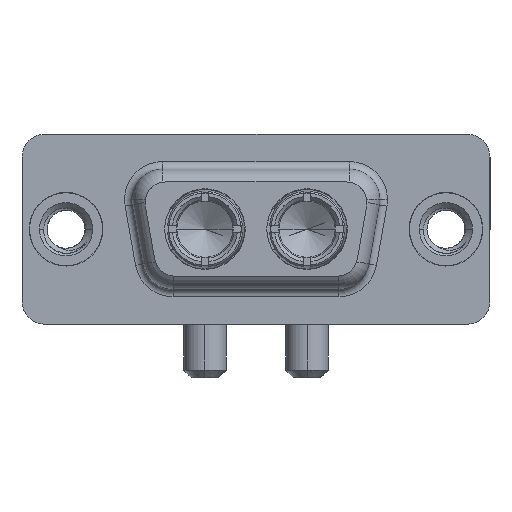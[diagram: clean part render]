
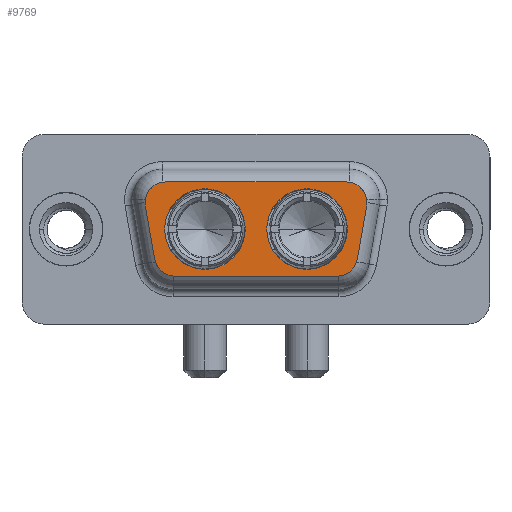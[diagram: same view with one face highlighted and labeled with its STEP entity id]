
A CAD part, top view. The second image highlights one B-rep face of the part: STEP entity #9769.
In plain terms, the highlighted planar face has unit normal (0, 0, 1).
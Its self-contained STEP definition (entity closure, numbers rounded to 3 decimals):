
#40 = DIRECTION ( 'NONE',  ( 0.174, -0.985, 0. ) ) ;
#42 = EDGE_CURVE ( 'NONE', #5957, #405, #10001, .T. ) ;
#180 = DIRECTION ( 'NONE',  ( -1., 0., 0. ) ) ;
#302 = AXIS2_PLACEMENT_3D ( 'NONE', #5699, #8658, #4725 ) ;
#391 = AXIS2_PLACEMENT_3D ( 'NONE', #10388, #2899, #4603 ) ;
#405 = VERTEX_POINT ( 'NONE', #8874 ) ;
#406 = CARTESIAN_POINT ( 'NONE',  ( 5.838, -1.984, 6.2 ) ) ;
#421 = CARTESIAN_POINT ( 'NONE',  ( 6.49, 0., 6.2 ) ) ;
#430 = VERTEX_POINT ( 'NONE', #421 ) ;
#628 = DIRECTION ( 'NONE',  ( -1., 0., 0. ) ) ;
#633 = EDGE_CURVE ( 'NONE', #10722, #5175, #7628, .T. ) ;
#653 = CARTESIAN_POINT ( 'NONE',  ( 17.833, -3.1, 6.2 ) ) ;
#724 = ORIENTED_EDGE ( 'NONE', *, *, #11435, .F. ) ;
#856 = CARTESIAN_POINT ( 'NONE',  ( 15.86, 0., 6.2 ) ) ;
#863 = VERTEX_POINT ( 'NONE', #6084 ) ;
#885 = VERTEX_POINT ( 'NONE', #406 ) ;
#1068 = DIRECTION ( 'NONE',  ( 0., 0., 1. ) ) ;
#1142 = VECTOR ( 'NONE', #3332, 1000. ) ;
#1339 = CIRCLE ( 'NONE', #9155, 1.35 ) ;
#1358 = ORIENTED_EDGE ( 'NONE', *, *, #3806, .T. ) ;
#1427 = LINE ( 'NONE', #10664, #9747 ) ;
#1580 = LINE ( 'NONE', #5340, #1142 ) ;
#1646 = DIRECTION ( 'NONE',  ( 1., 0., 0. ) ) ;
#1678 = CARTESIAN_POINT ( 'NONE',  ( 7.167, -1.75, 6.2 ) ) ;
#1778 = DIRECTION ( 'NONE',  ( 0., 0., 1. ) ) ;
#1855 = EDGE_CURVE ( 'NONE', #11892, #7952, #1427, .T. ) ;
#1967 = CARTESIAN_POINT ( 'NONE',  ( 7.167, -1.75, 6.2 ) ) ;
#1995 = ORIENTED_EDGE ( 'NONE', *, *, #9292, .T. ) ;
#2154 = ORIENTED_EDGE ( 'NONE', *, *, #11271, .F. ) ;
#2359 = AXIS2_PLACEMENT_3D ( 'NONE', #856, #1778, #2805 ) ;
#2431 = ORIENTED_EDGE ( 'NONE', *, *, #6789, .T. ) ;
#2529 = PLANE ( 'NONE',  #8586 ) ;
#2542 = CARTESIAN_POINT ( 'NONE',  ( 9.14, 0., 6.2 ) ) ;
#2555 = CARTESIAN_POINT ( 'NONE',  ( 6.55, 1.75, 6.2 ) ) ;
#2789 = ORIENTED_EDGE ( 'NONE', *, *, #1855, .T. ) ;
#2805 = DIRECTION ( 'NONE',  ( 1., 0., 0. ) ) ;
#2842 = ORIENTED_EDGE ( 'NONE', *, *, #633, .T. ) ;
#2899 = DIRECTION ( 'NONE',  ( 0., 0., 1. ) ) ;
#3009 = CARTESIAN_POINT ( 'NONE',  ( 18.45, 1.75, 6.2 ) ) ;
#3094 = CIRCLE ( 'NONE', #12130, 1.35 ) ;
#3165 = CARTESIAN_POINT ( 'NONE',  ( 5.2, 1.75, 6.2 ) ) ;
#3190 = EDGE_CURVE ( 'NONE', #10426, #430, #6930, .T. ) ;
#3332 = DIRECTION ( 'NONE',  ( 0.174, 0.985, 0. ) ) ;
#3621 = ORIENTED_EDGE ( 'NONE', *, *, #6040, .T. ) ;
#3806 = EDGE_CURVE ( 'NONE', #7587, #6211, #8054, .T. ) ;
#3811 = VERTEX_POINT ( 'NONE', #9425 ) ;
#3842 = CIRCLE ( 'NONE', #4412, 1.35 ) ;
#3971 = DIRECTION ( 'NONE',  ( -1., 0., 0. ) ) ;
#4228 = DIRECTION ( 'NONE',  ( -1., 0., 0. ) ) ;
#4288 = CIRCLE ( 'NONE', #391, 2.65 ) ;
#4338 = EDGE_CURVE ( 'NONE', #5175, #885, #6574, .T. ) ;
#4412 = AXIS2_PLACEMENT_3D ( 'NONE', #3009, #1068, #6734 ) ;
#4603 = DIRECTION ( 'NONE',  ( 1., 0., 0. ) ) ;
#4613 = VECTOR ( 'NONE', #40, 1000. ) ;
#4725 = DIRECTION ( 'NONE',  ( 1., 0., 0. ) ) ;
#5147 = DIRECTION ( 'NONE',  ( 0., 0., -1. ) ) ;
#5175 = VERTEX_POINT ( 'NONE', #6604 ) ;
#5317 = CARTESIAN_POINT ( 'NONE',  ( 11.79, 0., 6.2 ) ) ;
#5340 = CARTESIAN_POINT ( 'NONE',  ( 19.779, 1.516, 6.2 ) ) ;
#5606 = AXIS2_PLACEMENT_3D ( 'NONE', #7768, #11647, #10721 ) ;
#5682 = DIRECTION ( 'NONE',  ( 0., 0., 1. ) ) ;
#5699 = CARTESIAN_POINT ( 'NONE',  ( 9.14, 0., 6.2 ) ) ;
#5883 = ORIENTED_EDGE ( 'NONE', *, *, #4338, .T. ) ;
#5957 = VERTEX_POINT ( 'NONE', #11929 ) ;
#6040 = EDGE_CURVE ( 'NONE', #3811, #11892, #3842, .T. ) ;
#6084 = CARTESIAN_POINT ( 'NONE',  ( 19.162, -1.984, 6.2 ) ) ;
#6195 = CIRCLE ( 'NONE', #5606, 1.35 ) ;
#6211 = VERTEX_POINT ( 'NONE', #7898 ) ;
#6278 = DIRECTION ( 'NONE',  ( 0., 0., 1. ) ) ;
#6574 = LINE ( 'NONE', #8494, #4613 ) ;
#6604 = CARTESIAN_POINT ( 'NONE',  ( 5.221, 1.516, 6.2 ) ) ;
#6734 = DIRECTION ( 'NONE',  ( -1., 0., 0. ) ) ;
#6789 = EDGE_CURVE ( 'NONE', #7952, #10722, #6195, .T. ) ;
#6930 = CIRCLE ( 'NONE', #302, 2.65 ) ;
#7163 = FACE_BOUND ( 'NONE', #10277, .T. ) ;
#7179 = EDGE_CURVE ( 'NONE', #885, #7587, #1339, .T. ) ;
#7528 = CARTESIAN_POINT ( 'NONE',  ( 18.45, 3.1, 6.2 ) ) ;
#7587 = VERTEX_POINT ( 'NONE', #8447 ) ;
#7628 = CIRCLE ( 'NONE', #9222, 1.35 ) ;
#7759 = ORIENTED_EDGE ( 'NONE', *, *, #7179, .T. ) ;
#7768 = CARTESIAN_POINT ( 'NONE',  ( 6.55, 1.75, 6.2 ) ) ;
#7801 = AXIS2_PLACEMENT_3D ( 'NONE', #2542, #10998, #9100 ) ;
#7898 = CARTESIAN_POINT ( 'NONE',  ( 17.833, -3.1, 6.2 ) ) ;
#7907 = FACE_OUTER_BOUND ( 'NONE', #11882, .T. ) ;
#7952 = VERTEX_POINT ( 'NONE', #9027 ) ;
#8054 = LINE ( 'NONE', #653, #10783 ) ;
#8337 = ORIENTED_EDGE ( 'NONE', *, *, #42, .F. ) ;
#8447 = CARTESIAN_POINT ( 'NONE',  ( 7.167, -3.1, 6.2 ) ) ;
#8494 = CARTESIAN_POINT ( 'NONE',  ( 5.838, -1.984, 6.2 ) ) ;
#8586 = AXIS2_PLACEMENT_3D ( 'NONE', #1678, #5147, #4228 ) ;
#8658 = DIRECTION ( 'NONE',  ( 0., 0., 1. ) ) ;
#8874 = CARTESIAN_POINT ( 'NONE',  ( 18.51, 0., 6.2 ) ) ;
#9027 = CARTESIAN_POINT ( 'NONE',  ( 6.55, 3.1, 6.2 ) ) ;
#9100 = DIRECTION ( 'NONE',  ( 1., 0., 0. ) ) ;
#9155 = AXIS2_PLACEMENT_3D ( 'NONE', #1967, #5682, #180 ) ;
#9222 = AXIS2_PLACEMENT_3D ( 'NONE', #2555, #6278, #1646 ) ;
#9262 = EDGE_LOOP ( 'NONE', ( #724, #8337 ) ) ;
#9292 = EDGE_CURVE ( 'NONE', #863, #3811, #1580, .T. ) ;
#9425 = CARTESIAN_POINT ( 'NONE',  ( 19.779, 1.516, 6.2 ) ) ;
#9747 = VECTOR ( 'NONE', #3971, 1000. ) ;
#9769 = ADVANCED_FACE ( 'NONE', ( #11923, #7163, #7907 ), #2529, .F. ) ;
#9832 = DIRECTION ( 'NONE',  ( 0., 0., 1. ) ) ;
#9977 = CIRCLE ( 'NONE', #7801, 2.65 ) ;
#10001 = CIRCLE ( 'NONE', #2359, 2.65 ) ;
#10277 = EDGE_LOOP ( 'NONE', ( #10929, #2154 ) ) ;
#10388 = CARTESIAN_POINT ( 'NONE',  ( 15.86, 0., 6.2 ) ) ;
#10414 = EDGE_CURVE ( 'NONE', #6211, #863, #3094, .T. ) ;
#10426 = VERTEX_POINT ( 'NONE', #5317 ) ;
#10664 = CARTESIAN_POINT ( 'NONE',  ( 6.55, 3.1, 6.2 ) ) ;
#10721 = DIRECTION ( 'NONE',  ( 1., 0., 0. ) ) ;
#10722 = VERTEX_POINT ( 'NONE', #3165 ) ;
#10783 = VECTOR ( 'NONE', #10939, 1000. ) ;
#10929 = ORIENTED_EDGE ( 'NONE', *, *, #3190, .F. ) ;
#10939 = DIRECTION ( 'NONE',  ( 1., 0., 0. ) ) ;
#10998 = DIRECTION ( 'NONE',  ( 0., 0., 1. ) ) ;
#11216 = ORIENTED_EDGE ( 'NONE', *, *, #10414, .T. ) ;
#11271 = EDGE_CURVE ( 'NONE', #430, #10426, #9977, .T. ) ;
#11435 = EDGE_CURVE ( 'NONE', #405, #5957, #4288, .T. ) ;
#11647 = DIRECTION ( 'NONE',  ( 0., 0., 1. ) ) ;
#11792 = CARTESIAN_POINT ( 'NONE',  ( 17.833, -1.75, 6.2 ) ) ;
#11882 = EDGE_LOOP ( 'NONE', ( #7759, #1358, #11216, #1995, #3621, #2789, #2431, #2842, #5883 ) ) ;
#11892 = VERTEX_POINT ( 'NONE', #7528 ) ;
#11923 = FACE_BOUND ( 'NONE', #9262, .T. ) ;
#11929 = CARTESIAN_POINT ( 'NONE',  ( 13.21, 0., 6.2 ) ) ;
#12130 = AXIS2_PLACEMENT_3D ( 'NONE', #11792, #9832, #628 ) ;
